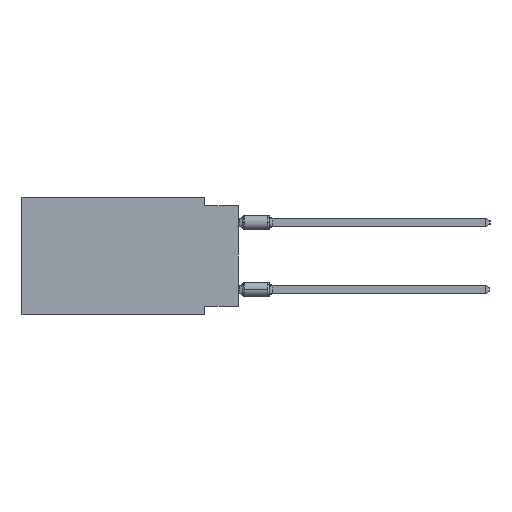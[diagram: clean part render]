
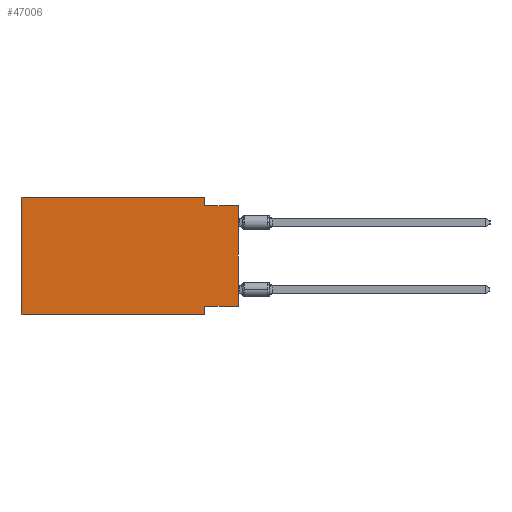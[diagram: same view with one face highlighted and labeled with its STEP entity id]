
A CAD part, left-side view. The second image highlights one B-rep face of the part: STEP entity #47006.
In plain terms, the highlighted planar face has unit normal (-1, 0, 0).
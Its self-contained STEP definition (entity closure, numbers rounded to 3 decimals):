
#4074 = EDGE_CURVE ( 'NONE', #38650, #20243, #44146, .T. ) ;
#4536 = VECTOR ( 'NONE', #12261, 1000. ) ;
#5318 = LINE ( 'NONE', #46992, #4536 ) ;
#5502 = CARTESIAN_POINT ( 'NONE',  ( 0., 2.54, -8.255 ) ) ;
#6324 = CARTESIAN_POINT ( 'NONE',  ( 0., 16.383, -8.89 ) ) ;
#7068 = EDGE_CURVE ( 'NONE', #25904, #20015, #5318, .T. ) ;
#8195 = EDGE_LOOP ( 'NONE', ( #18268, #31655, #8990, #31709, #41054, #43043, #11916, #24285 ) ) ;
#8626 = EDGE_CURVE ( 'NONE', #20243, #28549, #44979, .T. ) ;
#8990 = ORIENTED_EDGE ( 'NONE', *, *, #12771, .F. ) ;
#10160 = CARTESIAN_POINT ( 'NONE',  ( 0., 16.383, 0. ) ) ;
#10162 = DIRECTION ( 'NONE',  ( 0., 1., 0. ) ) ;
#11000 = CARTESIAN_POINT ( 'NONE',  ( 0., 2.54, -8.89 ) ) ;
#11292 = DIRECTION ( 'NONE',  ( 0., -1., 0. ) ) ;
#11504 = DIRECTION ( 'NONE',  ( 0., 0., -1. ) ) ;
#11602 = VECTOR ( 'NONE', #22666, 1000. ) ;
#11666 = EDGE_CURVE ( 'NONE', #20015, #44716, #23356, .T. ) ;
#11729 = DIRECTION ( 'NONE',  ( 0., 0., -1. ) ) ;
#11916 = ORIENTED_EDGE ( 'NONE', *, *, #8626, .F. ) ;
#12198 = DIRECTION ( 'NONE',  ( 0., -1., 0. ) ) ;
#12261 = DIRECTION ( 'NONE',  ( 0., 0., 1. ) ) ;
#12771 = EDGE_CURVE ( 'NONE', #44716, #15647, #41297, .T. ) ;
#12796 = EDGE_CURVE ( 'NONE', #38650, #28138, #15979, .T. ) ;
#15647 = VERTEX_POINT ( 'NONE', #30098 ) ;
#15979 = LINE ( 'NONE', #48989, #11602 ) ;
#17613 = DIRECTION ( 'NONE',  ( 0., 0., -1. ) ) ;
#18268 = ORIENTED_EDGE ( 'NONE', *, *, #12796, .T. ) ;
#19245 = LINE ( 'NONE', #34376, #22865 ) ;
#20015 = VERTEX_POINT ( 'NONE', #44537 ) ;
#20243 = VERTEX_POINT ( 'NONE', #5502 ) ;
#22290 = FACE_OUTER_BOUND ( 'NONE', #8195, .T. ) ;
#22666 = DIRECTION ( 'NONE',  ( 0., 0., 1. ) ) ;
#22696 = LINE ( 'NONE', #48766, #41085 ) ;
#22865 = VECTOR ( 'NONE', #22971, 1000. ) ;
#22971 = DIRECTION ( 'NONE',  ( 0., -1., 0. ) ) ;
#23220 = EDGE_CURVE ( 'NONE', #15647, #28138, #19245, .T. ) ;
#23356 = LINE ( 'NONE', #38762, #33454 ) ;
#24285 = ORIENTED_EDGE ( 'NONE', *, *, #4074, .F. ) ;
#25312 = CARTESIAN_POINT ( 'NONE',  ( 0., 0., -0.635 ) ) ;
#25904 = VERTEX_POINT ( 'NONE', #6324 ) ;
#26662 = VECTOR ( 'NONE', #11504, 1000. ) ;
#27713 = AXIS2_PLACEMENT_3D ( 'NONE', #10160, #32732, #17613 ) ;
#28138 = VERTEX_POINT ( 'NONE', #25312 ) ;
#28549 = VERTEX_POINT ( 'NONE', #46501 ) ;
#30098 = CARTESIAN_POINT ( 'NONE',  ( 0., 2.54, -0.635 ) ) ;
#31655 = ORIENTED_EDGE ( 'NONE', *, *, #23220, .F. ) ;
#31709 = ORIENTED_EDGE ( 'NONE', *, *, #11666, .F. ) ;
#32732 = DIRECTION ( 'NONE',  ( 1., 0., 0. ) ) ;
#32838 = CARTESIAN_POINT ( 'NONE',  ( 0., 0., -8.255 ) ) ;
#33454 = VECTOR ( 'NONE', #12198, 1000. ) ;
#34376 = CARTESIAN_POINT ( 'NONE',  ( 0., 0., -0.635 ) ) ;
#36699 = PLANE ( 'NONE',  #27713 ) ;
#37120 = VECTOR ( 'NONE', #11729, 1000. ) ;
#38650 = VERTEX_POINT ( 'NONE', #32838 ) ;
#38762 = CARTESIAN_POINT ( 'NONE',  ( 0., 16.383, 0. ) ) ;
#39935 = CARTESIAN_POINT ( 'NONE',  ( 0., 0., -8.255 ) ) ;
#41054 = ORIENTED_EDGE ( 'NONE', *, *, #7068, .F. ) ;
#41085 = VECTOR ( 'NONE', #11292, 1000. ) ;
#41297 = LINE ( 'NONE', #45255, #26662 ) ;
#43043 = ORIENTED_EDGE ( 'NONE', *, *, #45811, .T. ) ;
#44146 = LINE ( 'NONE', #39935, #46425 ) ;
#44537 = CARTESIAN_POINT ( 'NONE',  ( 0., 16.383, 0. ) ) ;
#44716 = VERTEX_POINT ( 'NONE', #46496 ) ;
#44979 = LINE ( 'NONE', #11000, #37120 ) ;
#45255 = CARTESIAN_POINT ( 'NONE',  ( 0., 2.54, 0. ) ) ;
#45811 = EDGE_CURVE ( 'NONE', #25904, #28549, #22696, .T. ) ;
#46425 = VECTOR ( 'NONE', #10162, 1000. ) ;
#46496 = CARTESIAN_POINT ( 'NONE',  ( 0., 2.54, 0. ) ) ;
#46501 = CARTESIAN_POINT ( 'NONE',  ( 0., 2.54, -8.89 ) ) ;
#46992 = CARTESIAN_POINT ( 'NONE',  ( 0., 16.383, 0. ) ) ;
#47006 = ADVANCED_FACE ( 'NONE', ( #22290 ), #36699, .F. ) ;
#48766 = CARTESIAN_POINT ( 'NONE',  ( 0., 16.383, -8.89 ) ) ;
#48989 = CARTESIAN_POINT ( 'NONE',  ( 0., 0., 0. ) ) ;
